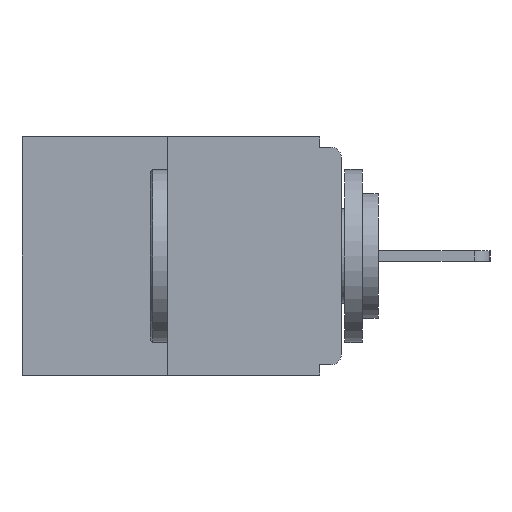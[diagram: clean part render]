
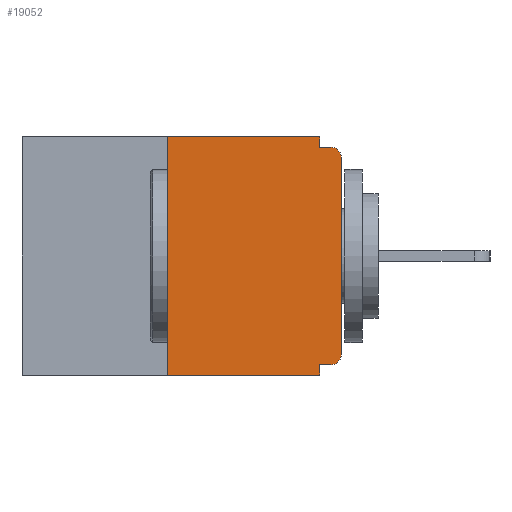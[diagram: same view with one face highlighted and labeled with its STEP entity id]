
A CAD part, left-side view. The second image highlights one B-rep face of the part: STEP entity #19052.
In plain terms, the highlighted planar face has unit normal (-1, 0, 0).
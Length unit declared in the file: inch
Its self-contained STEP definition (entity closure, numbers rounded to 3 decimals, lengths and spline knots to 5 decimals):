
#290 = DIRECTION ( 'NONE',  ( 1., 0., 0. ) ) ;
#427 = CARTESIAN_POINT ( 'NONE',  ( 0., 0.25, 0. ) ) ;
#635 = AXIS2_PLACEMENT_3D ( 'NONE', #7211, #21483, #9275 ) ;
#1173 = ORIENTED_EDGE ( 'NONE', *, *, #22361, .F. ) ;
#1194 = LINE ( 'NONE', #6802, #22436 ) ;
#1394 = CARTESIAN_POINT ( 'NONE',  ( 0., 0.031, -0.343 ) ) ;
#1860 = CARTESIAN_POINT ( 'NONE',  ( 0., 0., -0.03 ) ) ;
#2426 = EDGE_CURVE ( 'NONE', #15775, #19204, #5827, .T. ) ;
#4098 = LINE ( 'NONE', #20262, #23853 ) ;
#4502 = CARTESIAN_POINT ( 'NONE',  ( 0., 0.46, 0. ) ) ;
#5319 = VECTOR ( 'NONE', #9461, 39.37008 ) ;
#5487 = ORIENTED_EDGE ( 'NONE', *, *, #18176, .T. ) ;
#5695 = CIRCLE ( 'NONE', #635, 0.015 ) ;
#5753 = VERTEX_POINT ( 'NONE', #9626 ) ;
#5827 = LINE ( 'NONE', #25821, #21497 ) ;
#5859 = DIRECTION ( 'NONE',  ( 0., 0., -1. ) ) ;
#5933 = DIRECTION ( 'NONE',  ( -1., 0., 0. ) ) ;
#6796 = DIRECTION ( 'NONE',  ( 0., 0., 1. ) ) ;
#6802 = CARTESIAN_POINT ( 'NONE',  ( 0., 0.25, 0. ) ) ;
#7211 = CARTESIAN_POINT ( 'NONE',  ( 0., 0.015, -0.313 ) ) ;
#7556 = VERTEX_POINT ( 'NONE', #15957 ) ;
#7704 = CARTESIAN_POINT ( 'NONE',  ( 0., 0.25, -0.343 ) ) ;
#8012 = DIRECTION ( 'NONE',  ( 0., -1., 0. ) ) ;
#8152 = VERTEX_POINT ( 'NONE', #7704 ) ;
#8168 = FACE_OUTER_BOUND ( 'NONE', #14174, .T. ) ;
#8236 = EDGE_CURVE ( 'NONE', #8152, #25160, #1194, .T. ) ;
#8428 = ORIENTED_EDGE ( 'NONE', *, *, #26305, .T. ) ;
#9275 = DIRECTION ( 'NONE',  ( 0., 0., -1. ) ) ;
#9461 = DIRECTION ( 'NONE',  ( 0., 1., 0. ) ) ;
#9505 = CARTESIAN_POINT ( 'NONE',  ( 0., 0.031, -0.343 ) ) ;
#9626 = CARTESIAN_POINT ( 'NONE',  ( 0., 0., -0.313 ) ) ;
#9707 = ORIENTED_EDGE ( 'NONE', *, *, #20902, .T. ) ;
#9708 = LINE ( 'NONE', #1394, #19958 ) ;
#10002 = CARTESIAN_POINT ( 'NONE',  ( 0., 0.031, 0. ) ) ;
#10613 = CARTESIAN_POINT ( 'NONE',  ( 0., 0.031, -0.015 ) ) ;
#11526 = CARTESIAN_POINT ( 'NONE',  ( 0., 0., -0.328 ) ) ;
#11987 = VECTOR ( 'NONE', #25614, 39.37008 ) ;
#12349 = CARTESIAN_POINT ( 'NONE',  ( 0., 0.031, -0.328 ) ) ;
#12688 = AXIS2_PLACEMENT_3D ( 'NONE', #4502, #290, #14852 ) ;
#12827 = PLANE ( 'NONE',  #12688 ) ;
#13246 = ORIENTED_EDGE ( 'NONE', *, *, #8236, .F. ) ;
#13587 = EDGE_CURVE ( 'NONE', #7556, #25010, #15614, .T. ) ;
#13696 = LINE ( 'NONE', #19189, #19096 ) ;
#14080 = EDGE_CURVE ( 'NONE', #25160, #14635, #13696, .T. ) ;
#14174 = EDGE_LOOP ( 'NONE', ( #23301, #13246, #8428, #19305, #19956, #9707, #20594, #5487, #21813, #1173 ) ) ;
#14635 = VERTEX_POINT ( 'NONE', #19175 ) ;
#14852 = DIRECTION ( 'NONE',  ( 0., 0., -1. ) ) ;
#15385 = CARTESIAN_POINT ( 'NONE',  ( 0., 0.015, -0.015 ) ) ;
#15614 = LINE ( 'NONE', #11526, #5319 ) ;
#15775 = VERTEX_POINT ( 'NONE', #10613 ) ;
#15957 = CARTESIAN_POINT ( 'NONE',  ( 0., 0.015, -0.328 ) ) ;
#18176 = EDGE_CURVE ( 'NONE', #22424, #19204, #24337, .T. ) ;
#18222 = CARTESIAN_POINT ( 'NONE',  ( 0., 0.015, -0.03 ) ) ;
#18323 = AXIS2_PLACEMENT_3D ( 'NONE', #18222, #5933, #20290 ) ;
#19052 = ADVANCED_FACE ( 'NONE', ( #8168 ), #12827, .F. ) ;
#19096 = VECTOR ( 'NONE', #21217, 39.37008 ) ;
#19175 = CARTESIAN_POINT ( 'NONE',  ( 0., 0.031, 0. ) ) ;
#19189 = CARTESIAN_POINT ( 'NONE',  ( 0., 0.46, 0. ) ) ;
#19204 = VERTEX_POINT ( 'NONE', #15385 ) ;
#19305 = ORIENTED_EDGE ( 'NONE', *, *, #24957, .F. ) ;
#19853 = DIRECTION ( 'NONE',  ( 0., 0., -1. ) ) ;
#19956 = ORIENTED_EDGE ( 'NONE', *, *, #13587, .F. ) ;
#19958 = VECTOR ( 'NONE', #19853, 39.37008 ) ;
#20262 = CARTESIAN_POINT ( 'NONE',  ( 0., 0.46, -0.343 ) ) ;
#20290 = DIRECTION ( 'NONE',  ( 0., 0., -1. ) ) ;
#20416 = EDGE_CURVE ( 'NONE', #5753, #22424, #22736, .T. ) ;
#20594 = ORIENTED_EDGE ( 'NONE', *, *, #20416, .T. ) ;
#20902 = EDGE_CURVE ( 'NONE', #7556, #5753, #5695, .T. ) ;
#21001 = LINE ( 'NONE', #10002, #26201 ) ;
#21217 = DIRECTION ( 'NONE',  ( 0., -1., 0. ) ) ;
#21483 = DIRECTION ( 'NONE',  ( -1., 0., 0. ) ) ;
#21497 = VECTOR ( 'NONE', #26070, 39.37008 ) ;
#21547 = VERTEX_POINT ( 'NONE', #9505 ) ;
#21813 = ORIENTED_EDGE ( 'NONE', *, *, #2426, .F. ) ;
#22361 = EDGE_CURVE ( 'NONE', #14635, #15775, #21001, .T. ) ;
#22424 = VERTEX_POINT ( 'NONE', #1860 ) ;
#22436 = VECTOR ( 'NONE', #6796, 39.37008 ) ;
#22736 = LINE ( 'NONE', #23709, #11987 ) ;
#23301 = ORIENTED_EDGE ( 'NONE', *, *, #14080, .F. ) ;
#23709 = CARTESIAN_POINT ( 'NONE',  ( 0., 0., 0. ) ) ;
#23853 = VECTOR ( 'NONE', #8012, 39.37008 ) ;
#24337 = CIRCLE ( 'NONE', #18323, 0.015 ) ;
#24957 = EDGE_CURVE ( 'NONE', #25010, #21547, #9708, .T. ) ;
#25010 = VERTEX_POINT ( 'NONE', #12349 ) ;
#25160 = VERTEX_POINT ( 'NONE', #427 ) ;
#25614 = DIRECTION ( 'NONE',  ( 0., 0., 1. ) ) ;
#25821 = CARTESIAN_POINT ( 'NONE',  ( 0., 0., -0.015 ) ) ;
#26070 = DIRECTION ( 'NONE',  ( 0., -1., 0. ) ) ;
#26201 = VECTOR ( 'NONE', #5859, 39.37008 ) ;
#26305 = EDGE_CURVE ( 'NONE', #8152, #21547, #4098, .T. ) ;
